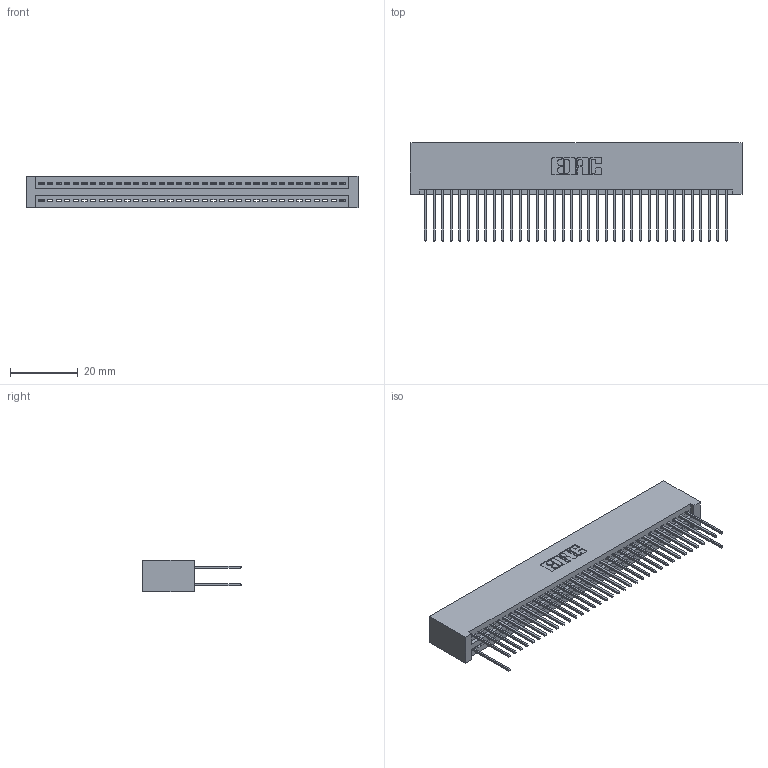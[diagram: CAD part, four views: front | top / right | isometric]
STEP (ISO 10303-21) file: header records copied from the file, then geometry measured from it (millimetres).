
FILE_DESCRIPTION (( 'STEP AP203' ), '1' );
FILE_NAME ('395-072-540-201.STEP', '2018-11-27T10:48:46', ( '' ), ( '' ), 'SwSTEP 2.0', 'SolidWorks 2016', '' );
FILE_SCHEMA (( 'CONFIG_CONTROL_DESIGN' ));
Length unit declared in the file: inch
Products named in the file (3): 395-072-540-201; 345-292-001_345-293-140; 345 Part_No Mounting Lugs
Assembly tree (39 placements, depth 2):
  395-072-540-201
    345 Part_No Mounting Lugs
    345-292-001_345-293-140  x38
Bounding box: 98.04 x 29.13 x 9.4 mm (x, y, z)
Volume: 9921.9 mm3; surface area: 13785.8 mm2
Topology: 39 solids, 39 shells, 2290 faces, 6897 edges, 4546 vertices
Faces by surface type: plane 1568, cylinder 722
Entity records: 27707 total; most frequent: CARTESIAN_POINT 4798, ORIENTED_EDGE 4766, DIRECTION 4195, EDGE_CURVE 2383, VECTOR 2115, LINE 2115, VERTEX_POINT 1586, AXIS2_PLACEMENT_3D 1040
